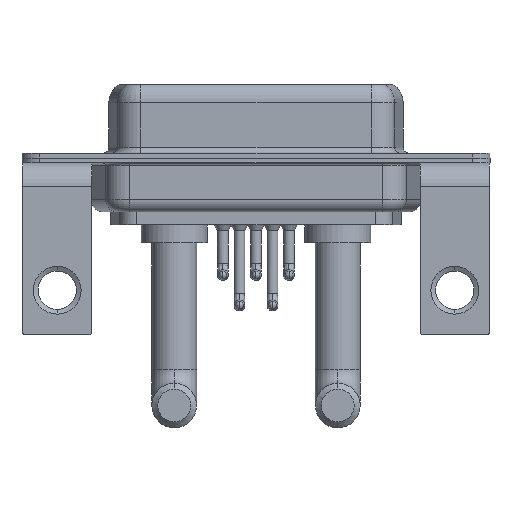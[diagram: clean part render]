
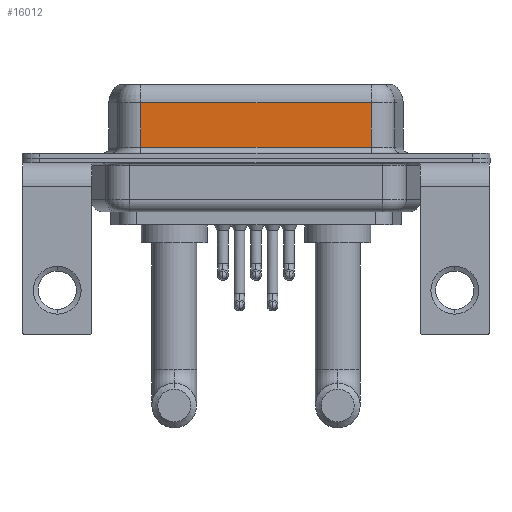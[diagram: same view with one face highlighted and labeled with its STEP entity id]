
A CAD part, front view. The second image highlights one B-rep face of the part: STEP entity #16012.
In plain terms, the highlighted planar face has unit normal (0, -1, 0).
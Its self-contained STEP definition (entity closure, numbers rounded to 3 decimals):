
#1 = VERTEX_POINT ( 'NONE', #15980 ) ;
#329 = ORIENTED_EDGE ( 'NONE', *, *, #12764, .T. ) ;
#965 = CARTESIAN_POINT ( 'NONE',  ( 26.287, -3.95, 0.9 ) ) ;
#1453 = PLANE ( 'NONE',  #8518 ) ;
#1532 = CARTESIAN_POINT ( 'NONE',  ( 26.287, -3.95, 6.4 ) ) ;
#2217 = EDGE_CURVE ( 'NONE', #11120, #1, #17567, .T. ) ;
#2696 = CARTESIAN_POINT ( 'NONE',  ( 26.287, -3.95, 6.4 ) ) ;
#3844 = CARTESIAN_POINT ( 'NONE',  ( 7.013, -3.95, 6.4 ) ) ;
#4338 = CARTESIAN_POINT ( 'NONE',  ( 7.013, -3.95, 4.65 ) ) ;
#4394 = DIRECTION ( 'NONE',  ( 0., 0., 1. ) ) ;
#6343 = ORIENTED_EDGE ( 'NONE', *, *, #2217, .T. ) ;
#8095 = LINE ( 'NONE', #13728, #15542 ) ;
#8155 = DIRECTION ( 'NONE',  ( 0., 0., -1. ) ) ;
#8393 = VERTEX_POINT ( 'NONE', #965 ) ;
#8518 = AXIS2_PLACEMENT_3D ( 'NONE', #1532, #15197, #4394 ) ;
#9553 = DIRECTION ( 'NONE',  ( -1., 0., 0. ) ) ;
#9598 = DIRECTION ( 'NONE',  ( 1., 0., 0. ) ) ;
#9991 = VECTOR ( 'NONE', #8155, 1000. ) ;
#11014 = FACE_OUTER_BOUND ( 'NONE', #11236, .T. ) ;
#11120 = VERTEX_POINT ( 'NONE', #4338 ) ;
#11170 = ORIENTED_EDGE ( 'NONE', *, *, #13060, .T. ) ;
#11236 = EDGE_LOOP ( 'NONE', ( #15383, #11170, #6343, #329 ) ) ;
#11810 = LINE ( 'NONE', #13160, #17250 ) ;
#12162 = VECTOR ( 'NONE', #14735, 1000. ) ;
#12764 = EDGE_CURVE ( 'NONE', #1, #8393, #8095, .T. ) ;
#13060 = EDGE_CURVE ( 'NONE', #17105, #11120, #11810, .T. ) ;
#13160 = CARTESIAN_POINT ( 'NONE',  ( 26.287, -3.95, 4.65 ) ) ;
#13243 = CARTESIAN_POINT ( 'NONE',  ( 26.287, -3.95, 4.65 ) ) ;
#13728 = CARTESIAN_POINT ( 'NONE',  ( 26.287, -3.95, 0.9 ) ) ;
#14735 = DIRECTION ( 'NONE',  ( 0., 0., -1. ) ) ;
#14937 = LINE ( 'NONE', #2696, #9991 ) ;
#15197 = DIRECTION ( 'NONE',  ( 0., 1., 0. ) ) ;
#15383 = ORIENTED_EDGE ( 'NONE', *, *, #17299, .F. ) ;
#15542 = VECTOR ( 'NONE', #9598, 1000. ) ;
#15980 = CARTESIAN_POINT ( 'NONE',  ( 7.013, -3.95, 0.9 ) ) ;
#16012 = ADVANCED_FACE ( 'NONE', ( #11014 ), #1453, .F. ) ;
#17105 = VERTEX_POINT ( 'NONE', #13243 ) ;
#17250 = VECTOR ( 'NONE', #9553, 1000. ) ;
#17299 = EDGE_CURVE ( 'NONE', #17105, #8393, #14937, .T. ) ;
#17567 = LINE ( 'NONE', #3844, #12162 ) ;
